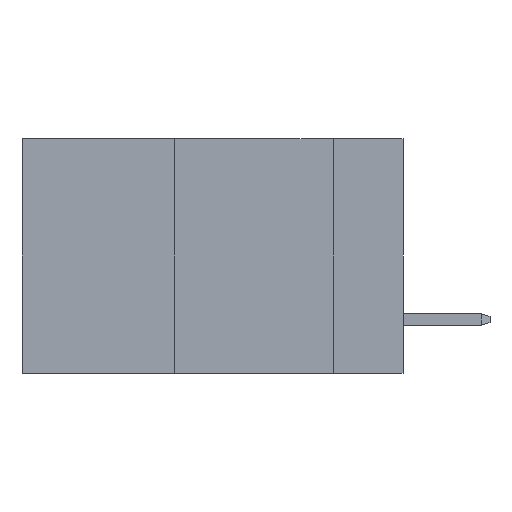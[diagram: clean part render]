
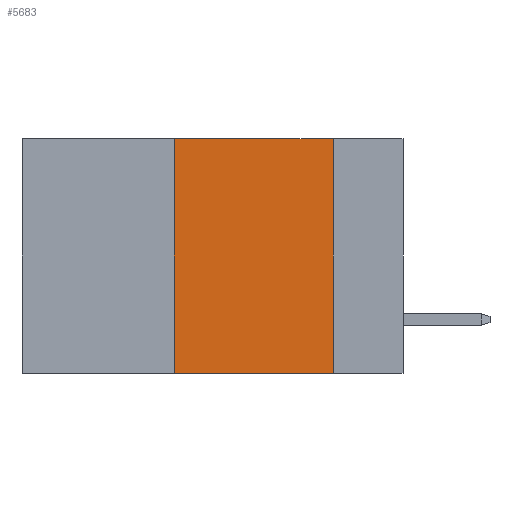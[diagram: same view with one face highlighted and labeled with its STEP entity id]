
A CAD part, left-side view. The second image highlights one B-rep face of the part: STEP entity #5683.
In plain terms, the highlighted planar face has unit normal (-1, 0, 0).
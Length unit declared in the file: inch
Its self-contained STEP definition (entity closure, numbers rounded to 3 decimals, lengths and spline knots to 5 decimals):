
#988 = ORIENTED_EDGE ( 'NONE', *, *, #9023, .F. ) ;
#1190 = DIRECTION ( 'NONE',  ( 0., 0., 1. ) ) ;
#1330 = CARTESIAN_POINT ( 'NONE',  ( 0., 0.11, -0.37 ) ) ;
#1684 = VERTEX_POINT ( 'NONE', #7697 ) ;
#1758 = CARTESIAN_POINT ( 'NONE',  ( 0., 0.6, 0. ) ) ;
#1832 = PLANE ( 'NONE',  #15494 ) ;
#2560 = VECTOR ( 'NONE', #2838, 39.37008 ) ;
#2592 = ORIENTED_EDGE ( 'NONE', *, *, #13542, .F. ) ;
#2838 = DIRECTION ( 'NONE',  ( 0., -1., 0. ) ) ;
#3303 = CARTESIAN_POINT ( 'NONE',  ( 0., 0.11, 0. ) ) ;
#3373 = EDGE_LOOP ( 'NONE', ( #14840, #2592, #988, #4266 ) ) ;
#4266 = ORIENTED_EDGE ( 'NONE', *, *, #13939, .T. ) ;
#4438 = DIRECTION ( 'NONE',  ( 0., -1., 0. ) ) ;
#5683 = ADVANCED_FACE ( 'NONE', ( #15512 ), #1832, .F. ) ;
#6468 = VECTOR ( 'NONE', #1190, 39.37008 ) ;
#6813 = CARTESIAN_POINT ( 'NONE',  ( 0., 0.6, 0. ) ) ;
#7697 = CARTESIAN_POINT ( 'NONE',  ( 0., 0.36, -0.37 ) ) ;
#7981 = EDGE_CURVE ( 'NONE', #13879, #12220, #13516, .T. ) ;
#8517 = VECTOR ( 'NONE', #12245, 39.37008 ) ;
#9023 = EDGE_CURVE ( 'NONE', #1684, #9371, #9948, .T. ) ;
#9185 = DIRECTION ( 'NONE',  ( 0., 0., -1. ) ) ;
#9371 = VERTEX_POINT ( 'NONE', #12680 ) ;
#9948 = LINE ( 'NONE', #15026, #6468 ) ;
#10237 = CARTESIAN_POINT ( 'NONE',  ( 0., 0.11, 0. ) ) ;
#10555 = LINE ( 'NONE', #10630, #12343 ) ;
#10630 = CARTESIAN_POINT ( 'NONE',  ( 0., 0.6, -0.37 ) ) ;
#11604 = DIRECTION ( 'NONE',  ( 1., 0., 0. ) ) ;
#12220 = VERTEX_POINT ( 'NONE', #1330 ) ;
#12245 = DIRECTION ( 'NONE',  ( 0., 0., -1. ) ) ;
#12343 = VECTOR ( 'NONE', #4438, 39.37008 ) ;
#12680 = CARTESIAN_POINT ( 'NONE',  ( 0., 0.36, 0. ) ) ;
#13516 = LINE ( 'NONE', #3303, #8517 ) ;
#13542 = EDGE_CURVE ( 'NONE', #9371, #13879, #14293, .T. ) ;
#13879 = VERTEX_POINT ( 'NONE', #10237 ) ;
#13939 = EDGE_CURVE ( 'NONE', #1684, #12220, #10555, .T. ) ;
#14293 = LINE ( 'NONE', #1758, #2560 ) ;
#14840 = ORIENTED_EDGE ( 'NONE', *, *, #7981, .F. ) ;
#15026 = CARTESIAN_POINT ( 'NONE',  ( 0., 0.36, 0. ) ) ;
#15494 = AXIS2_PLACEMENT_3D ( 'NONE', #6813, #11604, #9185 ) ;
#15512 = FACE_OUTER_BOUND ( 'NONE', #3373, .T. ) ;
